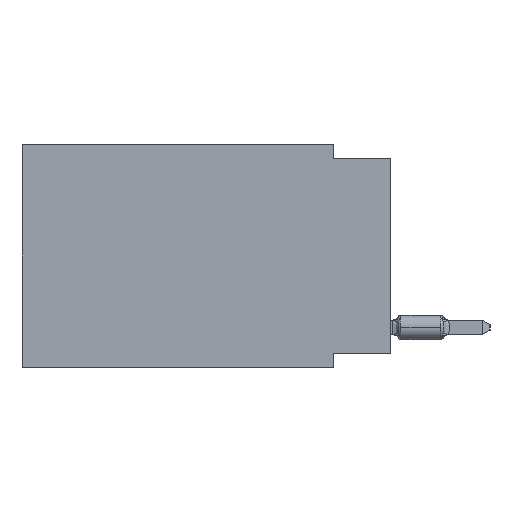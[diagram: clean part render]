
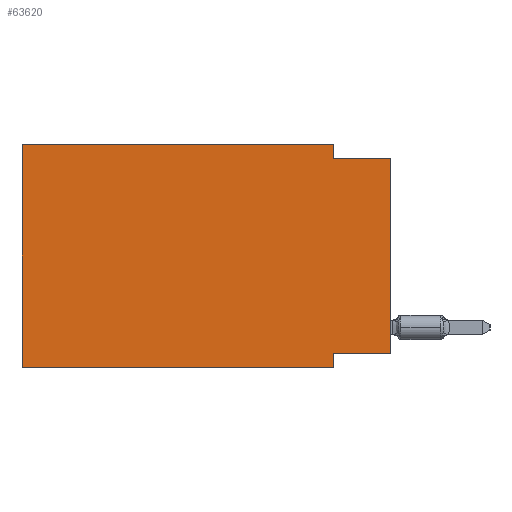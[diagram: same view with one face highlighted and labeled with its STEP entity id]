
A CAD part, left-side view. The second image highlights one B-rep face of the part: STEP entity #63620.
In plain terms, the highlighted planar face has unit normal (-1, 0, 0).
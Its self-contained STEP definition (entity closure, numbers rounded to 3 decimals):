
#1699 = VECTOR ( 'NONE', #61529, 1000. ) ;
#3466 = LINE ( 'NONE', #58906, #11206 ) ;
#4169 = VECTOR ( 'NONE', #37562, 1000. ) ;
#5749 = EDGE_CURVE ( 'NONE', #30898, #59188, #34222, .T. ) ;
#9931 = ORIENTED_EDGE ( 'NONE', *, *, #64912, .F. ) ;
#11206 = VECTOR ( 'NONE', #26260, 1000. ) ;
#13484 = LINE ( 'NONE', #24720, #33200 ) ;
#14919 = VERTEX_POINT ( 'NONE', #59398 ) ;
#18571 = DIRECTION ( 'NONE',  ( 0., -1., 0. ) ) ;
#18756 = LINE ( 'NONE', #40518, #40624 ) ;
#19418 = DIRECTION ( 'NONE',  ( 0., 0., -1. ) ) ;
#21052 = CARTESIAN_POINT ( 'NONE',  ( 0., 16.383, -9.906 ) ) ;
#21495 = EDGE_CURVE ( 'NONE', #52643, #61358, #26671, .T. ) ;
#21618 = CARTESIAN_POINT ( 'NONE',  ( 0., 2.54, 0. ) ) ;
#24720 = CARTESIAN_POINT ( 'NONE',  ( 0., 16.383, 0. ) ) ;
#25357 = VECTOR ( 'NONE', #49521, 1000. ) ;
#26260 = DIRECTION ( 'NONE',  ( 0., 0., -1. ) ) ;
#26312 = CARTESIAN_POINT ( 'NONE',  ( 0., 2.54, 0. ) ) ;
#26671 = LINE ( 'NONE', #26312, #25357 ) ;
#27823 = EDGE_LOOP ( 'NONE', ( #40265, #61386, #63824, #58467, #41333, #48198, #9931, #68873 ) ) ;
#28805 = CARTESIAN_POINT ( 'NONE',  ( 0., 16.383, -9.906 ) ) ;
#30139 = DIRECTION ( 'NONE',  ( 0., -1., 0. ) ) ;
#30898 = VERTEX_POINT ( 'NONE', #44499 ) ;
#33200 = VECTOR ( 'NONE', #18571, 1000. ) ;
#34004 = CARTESIAN_POINT ( 'NONE',  ( 0., 0., -9.271 ) ) ;
#34222 = LINE ( 'NONE', #56310, #64191 ) ;
#37562 = DIRECTION ( 'NONE',  ( 0., -1., 0. ) ) ;
#40265 = ORIENTED_EDGE ( 'NONE', *, *, #5749, .T. ) ;
#40518 = CARTESIAN_POINT ( 'NONE',  ( 0., 16.383, 0. ) ) ;
#40624 = VECTOR ( 'NONE', #63328, 1000. ) ;
#41150 = CARTESIAN_POINT ( 'NONE',  ( 0., 2.54, -0.635 ) ) ;
#41322 = VECTOR ( 'NONE', #30139, 1000. ) ;
#41333 = ORIENTED_EDGE ( 'NONE', *, *, #52499, .F. ) ;
#44024 = EDGE_CURVE ( 'NONE', #68021, #52643, #13484, .T. ) ;
#44499 = CARTESIAN_POINT ( 'NONE',  ( 0., 0., -9.271 ) ) ;
#44581 = EDGE_CURVE ( 'NONE', #61358, #59188, #60377, .T. ) ;
#45718 = CARTESIAN_POINT ( 'NONE',  ( 0., 16.383, 0. ) ) ;
#46281 = CARTESIAN_POINT ( 'NONE',  ( 0., 16.383, 0. ) ) ;
#46973 = VERTEX_POINT ( 'NONE', #21052 ) ;
#48198 = ORIENTED_EDGE ( 'NONE', *, *, #66362, .T. ) ;
#49521 = DIRECTION ( 'NONE',  ( 0., 0., -1. ) ) ;
#49948 = LINE ( 'NONE', #34004, #1699 ) ;
#50573 = LINE ( 'NONE', #28805, #41322 ) ;
#52416 = FACE_OUTER_BOUND ( 'NONE', #27823, .T. ) ;
#52499 = EDGE_CURVE ( 'NONE', #46973, #68021, #18756, .T. ) ;
#52643 = VERTEX_POINT ( 'NONE', #21618 ) ;
#55897 = EDGE_CURVE ( 'NONE', #30898, #14919, #49948, .T. ) ;
#56310 = CARTESIAN_POINT ( 'NONE',  ( 0., 0., 0. ) ) ;
#57475 = PLANE ( 'NONE',  #64251 ) ;
#58190 = DIRECTION ( 'NONE',  ( 1., 0., 0. ) ) ;
#58467 = ORIENTED_EDGE ( 'NONE', *, *, #44024, .F. ) ;
#58906 = CARTESIAN_POINT ( 'NONE',  ( 0., 2.54, -9.906 ) ) ;
#59188 = VERTEX_POINT ( 'NONE', #70348 ) ;
#59398 = CARTESIAN_POINT ( 'NONE',  ( 0., 2.54, -9.271 ) ) ;
#60377 = LINE ( 'NONE', #70203, #4169 ) ;
#61358 = VERTEX_POINT ( 'NONE', #41150 ) ;
#61386 = ORIENTED_EDGE ( 'NONE', *, *, #44581, .F. ) ;
#61529 = DIRECTION ( 'NONE',  ( 0., 1., 0. ) ) ;
#62082 = CARTESIAN_POINT ( 'NONE',  ( 0., 2.54, -9.906 ) ) ;
#63178 = DIRECTION ( 'NONE',  ( 0., 0., 1. ) ) ;
#63328 = DIRECTION ( 'NONE',  ( 0., 0., 1. ) ) ;
#63620 = ADVANCED_FACE ( 'NONE', ( #52416 ), #57475, .F. ) ;
#63824 = ORIENTED_EDGE ( 'NONE', *, *, #21495, .F. ) ;
#64191 = VECTOR ( 'NONE', #63178, 1000. ) ;
#64251 = AXIS2_PLACEMENT_3D ( 'NONE', #46281, #58190, #19418 ) ;
#64912 = EDGE_CURVE ( 'NONE', #14919, #67575, #3466, .T. ) ;
#66362 = EDGE_CURVE ( 'NONE', #46973, #67575, #50573, .T. ) ;
#67575 = VERTEX_POINT ( 'NONE', #62082 ) ;
#68021 = VERTEX_POINT ( 'NONE', #45718 ) ;
#68873 = ORIENTED_EDGE ( 'NONE', *, *, #55897, .F. ) ;
#70203 = CARTESIAN_POINT ( 'NONE',  ( 0., 0., -0.635 ) ) ;
#70348 = CARTESIAN_POINT ( 'NONE',  ( 0., 0., -0.635 ) ) ;
